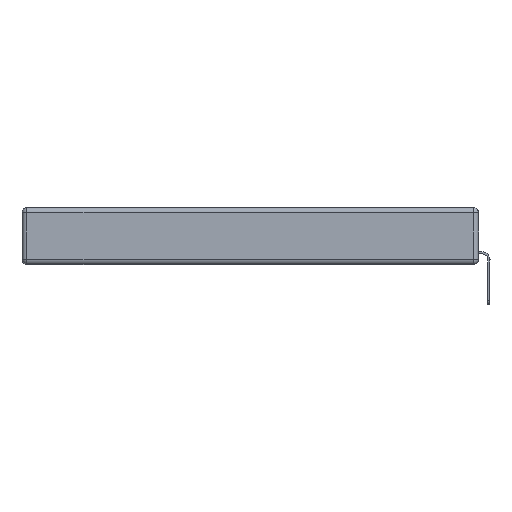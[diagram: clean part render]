
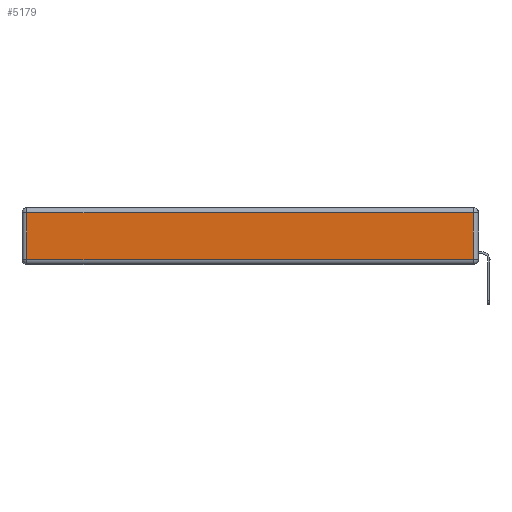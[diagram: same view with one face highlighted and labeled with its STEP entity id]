
A CAD part, left-side view. The second image highlights one B-rep face of the part: STEP entity #5179.
In plain terms, the highlighted planar face has unit normal (-1, 0, 0).
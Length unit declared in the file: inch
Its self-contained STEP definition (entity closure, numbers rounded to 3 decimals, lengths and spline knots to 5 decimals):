
#307 = EDGE_CURVE ( 'NONE', #11898, #5589, #3894, .T. ) ;
#692 = ORIENTED_EDGE ( 'NONE', *, *, #5058, .T. ) ;
#1132 = DIRECTION ( 'NONE',  ( 0., 0., 1. ) ) ;
#1263 = CARTESIAN_POINT ( 'NONE',  ( 0., 0., -0.313 ) ) ;
#1559 = FACE_OUTER_BOUND ( 'NONE', #10139, .T. ) ;
#2125 = LINE ( 'NONE', #11652, #7374 ) ;
#2568 = DIRECTION ( 'NONE',  ( 0., 1., 0. ) ) ;
#3032 = DIRECTION ( 'NONE',  ( 0., -1., 0. ) ) ;
#3894 = LINE ( 'NONE', #11840, #11525 ) ;
#5058 = EDGE_CURVE ( 'NONE', #7787, #5123, #2125, .T. ) ;
#5123 = VERTEX_POINT ( 'NONE', #8178 ) ;
#5179 = ADVANCED_FACE ( 'NONE', ( #1559 ), #9050, .T. ) ;
#5329 = CARTESIAN_POINT ( 'NONE',  ( 0., 0., -0.343 ) ) ;
#5498 = VECTOR ( 'NONE', #2568, 39.37008 ) ;
#5589 = VERTEX_POINT ( 'NONE', #8148 ) ;
#6352 = CARTESIAN_POINT ( 'NONE',  ( 0., 2.75, -0.03 ) ) ;
#7229 = ORIENTED_EDGE ( 'NONE', *, *, #7688, .T. ) ;
#7374 = VECTOR ( 'NONE', #9827, 39.37008 ) ;
#7688 = EDGE_CURVE ( 'NONE', #5589, #7787, #12022, .T. ) ;
#7715 = ORIENTED_EDGE ( 'NONE', *, *, #307, .T. ) ;
#7787 = VERTEX_POINT ( 'NONE', #9866 ) ;
#8148 = CARTESIAN_POINT ( 'NONE',  ( 0., 0.03, -0.03 ) ) ;
#8178 = CARTESIAN_POINT ( 'NONE',  ( 0., 2.72, -0.313 ) ) ;
#8236 = DIRECTION ( 'NONE',  ( 0., 0., 1. ) ) ;
#9050 = PLANE ( 'NONE',  #9178 ) ;
#9107 = VECTOR ( 'NONE', #3032, 39.37008 ) ;
#9178 = AXIS2_PLACEMENT_3D ( 'NONE', #5329, #9181, #8236 ) ;
#9181 = DIRECTION ( 'NONE',  ( -1., 0., 0. ) ) ;
#9656 = LINE ( 'NONE', #1263, #9107 ) ;
#9827 = DIRECTION ( 'NONE',  ( 0., 0., -1. ) ) ;
#9866 = CARTESIAN_POINT ( 'NONE',  ( 0., 2.72, -0.03 ) ) ;
#10131 = ORIENTED_EDGE ( 'NONE', *, *, #11571, .T. ) ;
#10139 = EDGE_LOOP ( 'NONE', ( #10131, #7715, #7229, #692 ) ) ;
#11005 = CARTESIAN_POINT ( 'NONE',  ( 0., 0.03, -0.313 ) ) ;
#11525 = VECTOR ( 'NONE', #1132, 39.37008 ) ;
#11571 = EDGE_CURVE ( 'NONE', #5123, #11898, #9656, .T. ) ;
#11652 = CARTESIAN_POINT ( 'NONE',  ( 0., 2.72, -0.343 ) ) ;
#11840 = CARTESIAN_POINT ( 'NONE',  ( 0., 0.03, -0.343 ) ) ;
#11898 = VERTEX_POINT ( 'NONE', #11005 ) ;
#12022 = LINE ( 'NONE', #6352, #5498 ) ;
